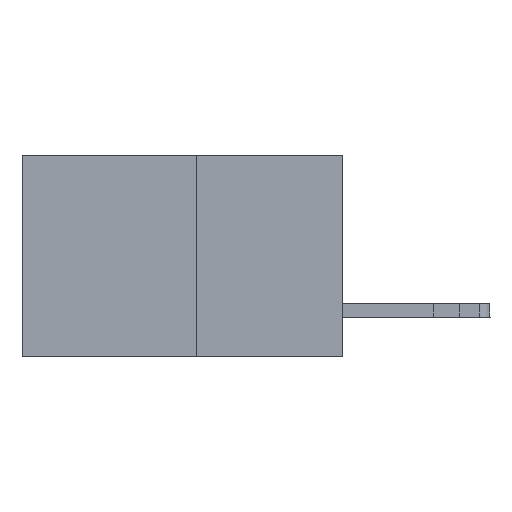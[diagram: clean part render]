
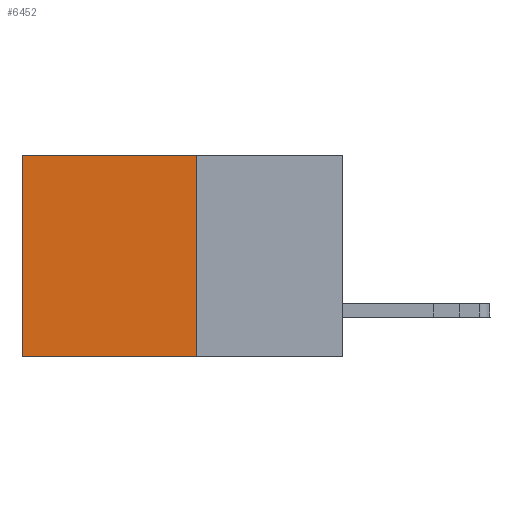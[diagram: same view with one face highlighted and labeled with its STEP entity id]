
A CAD part, left-side view. The second image highlights one B-rep face of the part: STEP entity #6452.
In plain terms, the highlighted planar face has unit normal (-1, 0, 0).
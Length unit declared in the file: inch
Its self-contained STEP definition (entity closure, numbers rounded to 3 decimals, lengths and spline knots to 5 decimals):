
#1548 = VECTOR ( 'NONE', #18220, 39.37008 ) ;
#1778 = CARTESIAN_POINT ( 'NONE',  ( 0.277, 0.27, 0. ) ) ;
#2259 = FACE_OUTER_BOUND ( 'NONE', #13640, .T. ) ;
#2739 = ORIENTED_EDGE ( 'NONE', *, *, #11291, .F. ) ;
#3219 = VECTOR ( 'NONE', #14090, 39.37008 ) ;
#3647 = CARTESIAN_POINT ( 'NONE',  ( 0.277, 0.27, -0.37 ) ) ;
#3654 = ORIENTED_EDGE ( 'NONE', *, *, #18210, .T. ) ;
#4959 = DIRECTION ( 'NONE',  ( 0., 1., 0. ) ) ;
#6093 = CARTESIAN_POINT ( 'NONE',  ( 0.277, 0.27, 0. ) ) ;
#6452 = ADVANCED_FACE ( 'NONE', ( #2259 ), #9536, .F. ) ;
#6648 = CARTESIAN_POINT ( 'NONE',  ( 0.277, 0.27, -0.37 ) ) ;
#7038 = CARTESIAN_POINT ( 'NONE',  ( 0.277, 0.59, -0.37 ) ) ;
#7221 = VERTEX_POINT ( 'NONE', #13879 ) ;
#7747 = VERTEX_POINT ( 'NONE', #6093 ) ;
#7921 = LINE ( 'NONE', #15475, #3219 ) ;
#8023 = AXIS2_PLACEMENT_3D ( 'NONE', #6648, #12626, #17302 ) ;
#8187 = VECTOR ( 'NONE', #4959, 39.37008 ) ;
#9536 = PLANE ( 'NONE',  #8023 ) ;
#9969 = CARTESIAN_POINT ( 'NONE',  ( 0.277, 0.27, -0.37 ) ) ;
#10194 = CARTESIAN_POINT ( 'NONE',  ( 0.277, 0.59, 0. ) ) ;
#10260 = LINE ( 'NONE', #9969, #17729 ) ;
#10368 = ORIENTED_EDGE ( 'NONE', *, *, #10999, .F. ) ;
#10999 = EDGE_CURVE ( 'NONE', #7747, #7221, #10260, .T. ) ;
#11242 = LINE ( 'NONE', #3647, #8187 ) ;
#11291 = EDGE_CURVE ( 'NONE', #7221, #17825, #11242, .T. ) ;
#12160 = LINE ( 'NONE', #1778, #1548 ) ;
#12626 = DIRECTION ( 'NONE',  ( 1., 0., 0. ) ) ;
#13640 = EDGE_LOOP ( 'NONE', ( #3654, #2739, #10368, #15975 ) ) ;
#13879 = CARTESIAN_POINT ( 'NONE',  ( 0.277, 0.27, -0.37 ) ) ;
#14090 = DIRECTION ( 'NONE',  ( 0., 0., -1. ) ) ;
#14781 = EDGE_CURVE ( 'NONE', #7747, #19511, #12160, .T. ) ;
#15475 = CARTESIAN_POINT ( 'NONE',  ( 0.277, 0.59, -0.37 ) ) ;
#15975 = ORIENTED_EDGE ( 'NONE', *, *, #14781, .T. ) ;
#17302 = DIRECTION ( 'NONE',  ( 0., 0., -1. ) ) ;
#17729 = VECTOR ( 'NONE', #19014, 39.37008 ) ;
#17825 = VERTEX_POINT ( 'NONE', #7038 ) ;
#18210 = EDGE_CURVE ( 'NONE', #19511, #17825, #7921, .T. ) ;
#18220 = DIRECTION ( 'NONE',  ( 0., 1., 0. ) ) ;
#19014 = DIRECTION ( 'NONE',  ( 0., 0., -1. ) ) ;
#19511 = VERTEX_POINT ( 'NONE', #10194 ) ;
